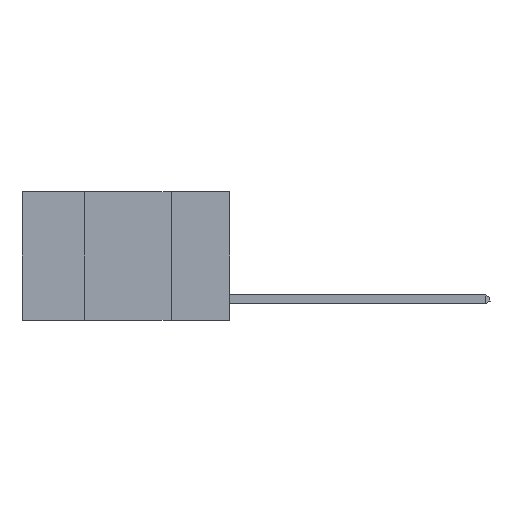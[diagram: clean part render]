
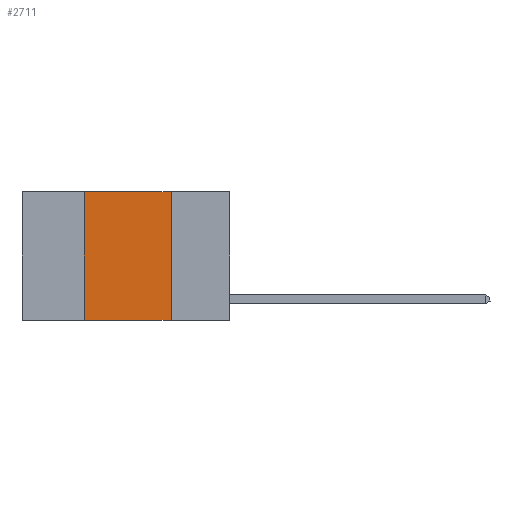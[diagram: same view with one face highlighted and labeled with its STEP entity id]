
A CAD part, left-side view. The second image highlights one B-rep face of the part: STEP entity #2711.
In plain terms, the highlighted planar face has unit normal (-1, 0, 0).
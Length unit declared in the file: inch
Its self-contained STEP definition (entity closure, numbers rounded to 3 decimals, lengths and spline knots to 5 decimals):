
#654 = AXIS2_PLACEMENT_3D ( 'NONE', #11037, #14214, #17095 ) ;
#2711 = ADVANCED_FACE ( 'NONE', ( #8441 ), #9539, .F. ) ;
#3149 = ORIENTED_EDGE ( 'NONE', *, *, #7420, .F. ) ;
#4488 = CARTESIAN_POINT ( 'NONE',  ( 0., 0.42, 0. ) ) ;
#4998 = LINE ( 'NONE', #11088, #15084 ) ;
#5195 = CARTESIAN_POINT ( 'NONE',  ( 0., 0.42, 0. ) ) ;
#5389 = VECTOR ( 'NONE', #18400, 39.37008 ) ;
#5598 = EDGE_CURVE ( 'NONE', #12741, #10049, #12494, .T. ) ;
#5602 = ORIENTED_EDGE ( 'NONE', *, *, #19199, .F. ) ;
#6517 = VECTOR ( 'NONE', #15947, 39.37008 ) ;
#7420 = EDGE_CURVE ( 'NONE', #19152, #13614, #4998, .T. ) ;
#7617 = ORIENTED_EDGE ( 'NONE', *, *, #5598, .T. ) ;
#8441 = FACE_OUTER_BOUND ( 'NONE', #8951, .T. ) ;
#8951 = EDGE_LOOP ( 'NONE', ( #5602, #3149, #14253, #7617 ) ) ;
#9360 = CARTESIAN_POINT ( 'NONE',  ( 0., 0.17, 0. ) ) ;
#9497 = LINE ( 'NONE', #5195, #15197 ) ;
#9539 = PLANE ( 'NONE',  #654 ) ;
#9591 = DIRECTION ( 'NONE',  ( 0., 0., 1. ) ) ;
#9677 = DIRECTION ( 'NONE',  ( 0., -1., 0. ) ) ;
#10049 = VERTEX_POINT ( 'NONE', #19116 ) ;
#10937 = CARTESIAN_POINT ( 'NONE',  ( 0., 0.17, 0. ) ) ;
#11037 = CARTESIAN_POINT ( 'NONE',  ( 0., 0.6, 0. ) ) ;
#11088 = CARTESIAN_POINT ( 'NONE',  ( 0., 0.6, 0. ) ) ;
#12494 = LINE ( 'NONE', #18924, #6517 ) ;
#12741 = VERTEX_POINT ( 'NONE', #12765 ) ;
#12765 = CARTESIAN_POINT ( 'NONE',  ( 0., 0.42, -0.37 ) ) ;
#13614 = VERTEX_POINT ( 'NONE', #10937 ) ;
#14214 = DIRECTION ( 'NONE',  ( 1., 0., 0. ) ) ;
#14253 = ORIENTED_EDGE ( 'NONE', *, *, #15719, .F. ) ;
#15084 = VECTOR ( 'NONE', #9677, 39.37008 ) ;
#15197 = VECTOR ( 'NONE', #9591, 39.37008 ) ;
#15719 = EDGE_CURVE ( 'NONE', #12741, #19152, #9497, .T. ) ;
#15947 = DIRECTION ( 'NONE',  ( 0., -1., 0. ) ) ;
#17095 = DIRECTION ( 'NONE',  ( 0., 0., -1. ) ) ;
#18202 = LINE ( 'NONE', #9360, #5389 ) ;
#18400 = DIRECTION ( 'NONE',  ( 0., 0., -1. ) ) ;
#18924 = CARTESIAN_POINT ( 'NONE',  ( 0., 0.6, -0.37 ) ) ;
#19116 = CARTESIAN_POINT ( 'NONE',  ( 0., 0.17, -0.37 ) ) ;
#19152 = VERTEX_POINT ( 'NONE', #4488 ) ;
#19199 = EDGE_CURVE ( 'NONE', #13614, #10049, #18202, .T. ) ;
